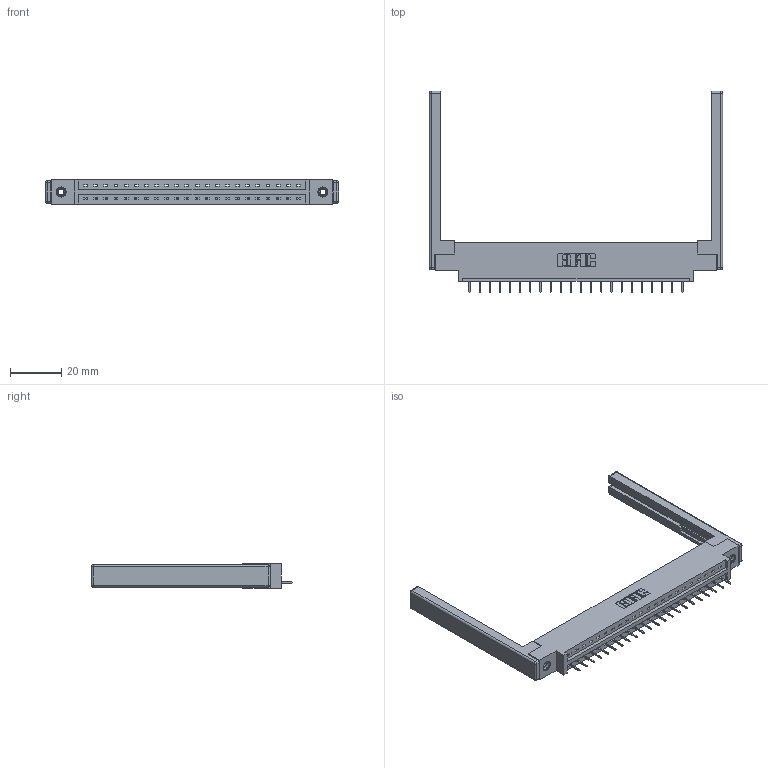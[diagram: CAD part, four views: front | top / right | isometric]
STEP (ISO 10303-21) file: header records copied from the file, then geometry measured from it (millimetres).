
FILE_DESCRIPTION (( 'STEP AP203' ), '1' );
FILE_NAME ('387-022-524-668.STEP', '2019-10-03T01:17:20', ( '' ), ( '' ), 'SwSTEP 2.0', 'SolidWorks 2016', '' );
FILE_SCHEMA (( 'CONFIG_CONTROL_DESIGN' ));
Length unit declared in the file: inch
Products named in the file (5): 345-292-001_345-293-124; 345-250-001_345-250-001-102; 337 Part_0.170 Offset - 0.156 Dia-TI; 307-220-068; 387-022-524-668
Assembly tree (27 placements, depth 2):
  387-022-524-668
    337 Part_0.170 Offset - 0.156 Dia-TI
    345-292-001_345-293-124  x22
    345-250-001_345-250-001-102  x2
    307-220-068  x2
Bounding box: 114.6 x 78.75 x 9.4 mm (x, y, z)
Volume: 15847.8 mm3; surface area: 15611.1 mm2
Topology: 27 solids, 27 shells, 1724 faces, 4937 edges, 3182 vertices
Faces by surface type: plane 1306, cylinder 394, cone 12, sphere 8, torus 4
Entity records: 21906 total; most frequent: CARTESIAN_POINT 3769, ORIENTED_EDGE 3716, DIRECTION 3288, EDGE_CURVE 1858, VECTOR 1684, LINE 1684, VERTEX_POINT 1226, AXIS2_PLACEMENT_3D 802
